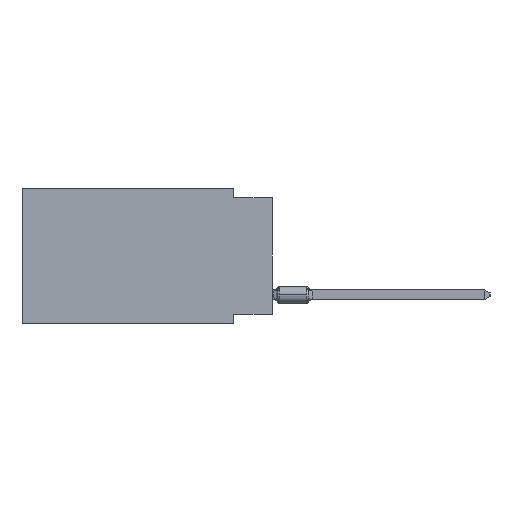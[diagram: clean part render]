
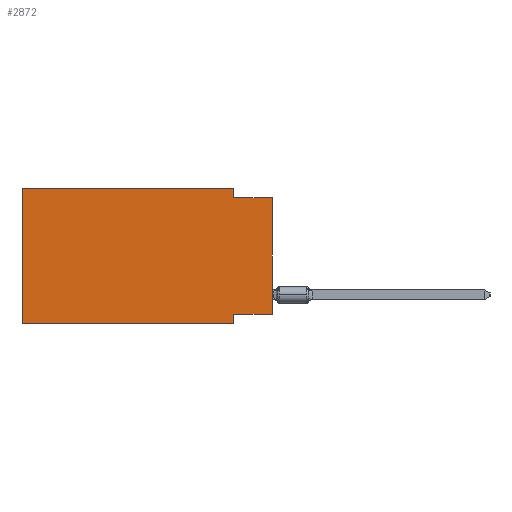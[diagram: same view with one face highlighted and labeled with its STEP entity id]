
A CAD part, left-side view. The second image highlights one B-rep face of the part: STEP entity #2872.
In plain terms, the highlighted planar face has unit normal (-1, 0, 0).
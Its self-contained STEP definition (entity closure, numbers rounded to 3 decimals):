
#607 = CARTESIAN_POINT ( 'NONE',  ( 0., 0., -0.635 ) ) ;
#688 = ORIENTED_EDGE ( 'NONE', *, *, #27941, .F. ) ;
#989 = CARTESIAN_POINT ( 'NONE',  ( 0., 16.383, -8.89 ) ) ;
#1289 = DIRECTION ( 'NONE',  ( 0., 0., -1. ) ) ;
#1414 = VERTEX_POINT ( 'NONE', #35224 ) ;
#2822 = VECTOR ( 'NONE', #19788, 1000. ) ;
#2872 = ADVANCED_FACE ( 'NONE', ( #31657 ), #3029, .F. ) ;
#3029 = PLANE ( 'NONE',  #29298 ) ;
#3313 = CARTESIAN_POINT ( 'NONE',  ( 0., 16.383, 0. ) ) ;
#4757 = LINE ( 'NONE', #17520, #5388 ) ;
#5078 = ORIENTED_EDGE ( 'NONE', *, *, #9956, .F. ) ;
#5286 = ORIENTED_EDGE ( 'NONE', *, *, #20194, .F. ) ;
#5388 = VECTOR ( 'NONE', #7495, 1000. ) ;
#6905 = VERTEX_POINT ( 'NONE', #989 ) ;
#7495 = DIRECTION ( 'NONE',  ( 0., 0., 1. ) ) ;
#9056 = EDGE_CURVE ( 'NONE', #19760, #21281, #16767, .T. ) ;
#9408 = ORIENTED_EDGE ( 'NONE', *, *, #31788, .F. ) ;
#9585 = EDGE_CURVE ( 'NONE', #1414, #33832, #32601, .T. ) ;
#9638 = CARTESIAN_POINT ( 'NONE',  ( 0., 0., 0. ) ) ;
#9743 = CARTESIAN_POINT ( 'NONE',  ( 0., 16.383, -8.89 ) ) ;
#9956 = EDGE_CURVE ( 'NONE', #30777, #19760, #33151, .T. ) ;
#10246 = VECTOR ( 'NONE', #1289, 1000. ) ;
#11820 = DIRECTION ( 'NONE',  ( 0., -1., 0. ) ) ;
#12091 = DIRECTION ( 'NONE',  ( 0., 0., -1. ) ) ;
#12162 = LINE ( 'NONE', #9638, #40255 ) ;
#12503 = LINE ( 'NONE', #15443, #23032 ) ;
#14048 = ORIENTED_EDGE ( 'NONE', *, *, #22054, .T. ) ;
#15443 = CARTESIAN_POINT ( 'NONE',  ( 0., 2.54, 0. ) ) ;
#15774 = CARTESIAN_POINT ( 'NONE',  ( 0., 16.383, 0. ) ) ;
#16767 = LINE ( 'NONE', #26580, #10246 ) ;
#17336 = DIRECTION ( 'NONE',  ( 0., -1., 0. ) ) ;
#17520 = CARTESIAN_POINT ( 'NONE',  ( 0., 16.383, 0. ) ) ;
#18512 = DIRECTION ( 'NONE',  ( 0., 0., -1. ) ) ;
#18906 = VECTOR ( 'NONE', #22712, 1000. ) ;
#19726 = CARTESIAN_POINT ( 'NONE',  ( 0., 2.54, -8.89 ) ) ;
#19760 = VERTEX_POINT ( 'NONE', #27157 ) ;
#19788 = DIRECTION ( 'NONE',  ( 0., -1., 0. ) ) ;
#19803 = CARTESIAN_POINT ( 'NONE',  ( 0., 0., -8.255 ) ) ;
#20018 = ORIENTED_EDGE ( 'NONE', *, *, #38368, .T. ) ;
#20194 = EDGE_CURVE ( 'NONE', #6905, #25447, #4757, .T. ) ;
#21281 = VERTEX_POINT ( 'NONE', #19726 ) ;
#21614 = VECTOR ( 'NONE', #17336, 1000. ) ;
#22054 = EDGE_CURVE ( 'NONE', #6905, #21281, #22914, .T. ) ;
#22091 = ORIENTED_EDGE ( 'NONE', *, *, #9056, .F. ) ;
#22712 = DIRECTION ( 'NONE',  ( 0., 1., 0. ) ) ;
#22914 = LINE ( 'NONE', #9743, #2822 ) ;
#23032 = VECTOR ( 'NONE', #12091, 1000. ) ;
#24515 = VECTOR ( 'NONE', #11820, 1000. ) ;
#25447 = VERTEX_POINT ( 'NONE', #3313 ) ;
#25858 = CARTESIAN_POINT ( 'NONE',  ( 0., 2.54, 0. ) ) ;
#26580 = CARTESIAN_POINT ( 'NONE',  ( 0., 2.54, -8.89 ) ) ;
#27157 = CARTESIAN_POINT ( 'NONE',  ( 0., 2.54, -8.255 ) ) ;
#27688 = LINE ( 'NONE', #33769, #24515 ) ;
#27941 = EDGE_CURVE ( 'NONE', #25447, #39189, #27688, .T. ) ;
#28460 = DIRECTION ( 'NONE',  ( 0., 0., 1. ) ) ;
#28514 = DIRECTION ( 'NONE',  ( 1., 0., 0. ) ) ;
#29298 = AXIS2_PLACEMENT_3D ( 'NONE', #15774, #28514, #18512 ) ;
#30777 = VERTEX_POINT ( 'NONE', #31497 ) ;
#31497 = CARTESIAN_POINT ( 'NONE',  ( 0., 0., -8.255 ) ) ;
#31657 = FACE_OUTER_BOUND ( 'NONE', #33936, .T. ) ;
#31788 = EDGE_CURVE ( 'NONE', #39189, #1414, #12503, .T. ) ;
#32095 = ORIENTED_EDGE ( 'NONE', *, *, #9585, .F. ) ;
#32601 = LINE ( 'NONE', #39271, #21614 ) ;
#33151 = LINE ( 'NONE', #19803, #18906 ) ;
#33769 = CARTESIAN_POINT ( 'NONE',  ( 0., 16.383, 0. ) ) ;
#33832 = VERTEX_POINT ( 'NONE', #607 ) ;
#33936 = EDGE_LOOP ( 'NONE', ( #20018, #32095, #9408, #688, #5286, #14048, #22091, #5078 ) ) ;
#35224 = CARTESIAN_POINT ( 'NONE',  ( 0., 2.54, -0.635 ) ) ;
#38368 = EDGE_CURVE ( 'NONE', #30777, #33832, #12162, .T. ) ;
#39189 = VERTEX_POINT ( 'NONE', #25858 ) ;
#39271 = CARTESIAN_POINT ( 'NONE',  ( 0., 0., -0.635 ) ) ;
#40255 = VECTOR ( 'NONE', #28460, 1000. ) ;
